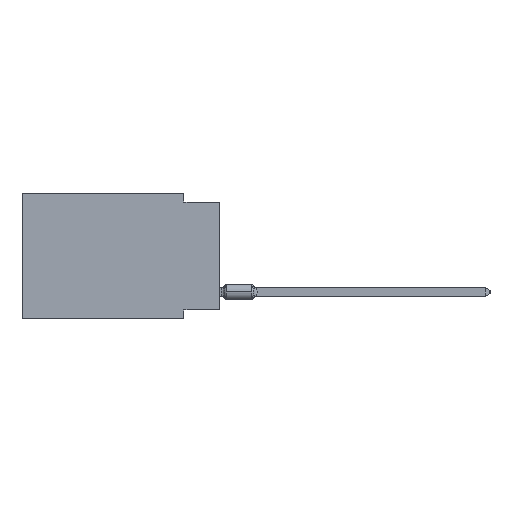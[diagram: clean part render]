
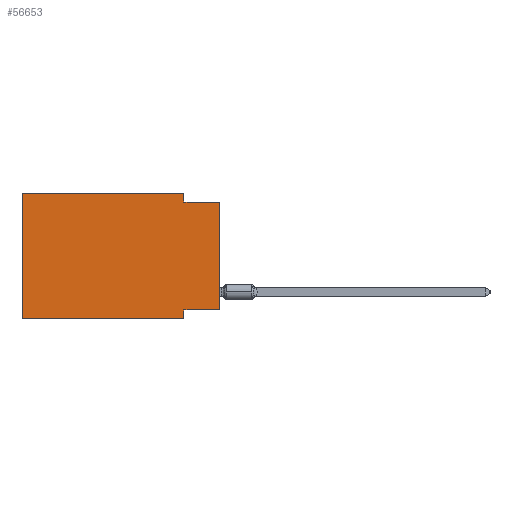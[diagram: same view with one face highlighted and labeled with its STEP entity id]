
A CAD part, left-side view. The second image highlights one B-rep face of the part: STEP entity #56653.
In plain terms, the highlighted planar face has unit normal (-1, 0, 0).
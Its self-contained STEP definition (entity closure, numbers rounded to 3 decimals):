
#1423 = ORIENTED_EDGE ( 'NONE', *, *, #35114, .F. ) ;
#5401 = CARTESIAN_POINT ( 'NONE',  ( 0., 13.97, 0. ) ) ;
#5918 = DIRECTION ( 'NONE',  ( 0., 0., 1. ) ) ;
#7233 = CARTESIAN_POINT ( 'NONE',  ( 0., 2.54, -8.255 ) ) ;
#7724 = LINE ( 'NONE', #23828, #65843 ) ;
#9683 = EDGE_CURVE ( 'NONE', #47627, #45161, #61070, .T. ) ;
#10409 = VERTEX_POINT ( 'NONE', #14607 ) ;
#11077 = ORIENTED_EDGE ( 'NONE', *, *, #18448, .F. ) ;
#14607 = CARTESIAN_POINT ( 'NONE',  ( 0., 0., -0.635 ) ) ;
#17439 = DIRECTION ( 'NONE',  ( 0., 0., 1. ) ) ;
#18448 = EDGE_CURVE ( 'NONE', #45444, #48281, #95899, .T. ) ;
#18705 = VECTOR ( 'NONE', #53018, 1000. ) ;
#22796 = CARTESIAN_POINT ( 'NONE',  ( 0., 2.54, -8.89 ) ) ;
#23828 = CARTESIAN_POINT ( 'NONE',  ( 0., 2.54, 0. ) ) ;
#24692 = VECTOR ( 'NONE', #36902, 1000. ) ;
#26858 = DIRECTION ( 'NONE',  ( 0., -1., 0. ) ) ;
#26885 = DIRECTION ( 'NONE',  ( 0., -1., 0. ) ) ;
#30345 = EDGE_CURVE ( 'NONE', #47627, #10409, #63252, .T. ) ;
#32315 = DIRECTION ( 'NONE',  ( 0., -1., 0. ) ) ;
#34377 = CARTESIAN_POINT ( 'NONE',  ( 0., 0., -0.635 ) ) ;
#35075 = VECTOR ( 'NONE', #26858, 1000. ) ;
#35114 = EDGE_CURVE ( 'NONE', #48281, #82652, #7724, .T. ) ;
#36902 = DIRECTION ( 'NONE',  ( 0., 1., 0. ) ) ;
#39866 = CARTESIAN_POINT ( 'NONE',  ( 0., 13.97, -8.89 ) ) ;
#41231 = ORIENTED_EDGE ( 'NONE', *, *, #56232, .T. ) ;
#42937 = VECTOR ( 'NONE', #17439, 1000. ) ;
#43924 = LINE ( 'NONE', #34377, #35075 ) ;
#45161 = VERTEX_POINT ( 'NONE', #7233 ) ;
#45444 = VERTEX_POINT ( 'NONE', #58999 ) ;
#47268 = ORIENTED_EDGE ( 'NONE', *, *, #9683, .F. ) ;
#47627 = VERTEX_POINT ( 'NONE', #49974 ) ;
#48281 = VERTEX_POINT ( 'NONE', #71784 ) ;
#49974 = CARTESIAN_POINT ( 'NONE',  ( 0., 0., -8.255 ) ) ;
#50646 = CARTESIAN_POINT ( 'NONE',  ( 0., 13.97, 0. ) ) ;
#53018 = DIRECTION ( 'NONE',  ( 0., 0., -1. ) ) ;
#53118 = CARTESIAN_POINT ( 'NONE',  ( 0., 13.97, -8.89 ) ) ;
#54215 = CARTESIAN_POINT ( 'NONE',  ( 0., 0., 0. ) ) ;
#56232 = EDGE_CURVE ( 'NONE', #90997, #75445, #63529, .T. ) ;
#56653 = ADVANCED_FACE ( 'NONE', ( #96994 ), #64756, .F. ) ;
#58999 = CARTESIAN_POINT ( 'NONE',  ( 0., 13.97, 0. ) ) ;
#59613 = ORIENTED_EDGE ( 'NONE', *, *, #30345, .T. ) ;
#60508 = ORIENTED_EDGE ( 'NONE', *, *, #86798, .F. ) ;
#61070 = LINE ( 'NONE', #89805, #24692 ) ;
#62747 = ORIENTED_EDGE ( 'NONE', *, *, #89873, .F. ) ;
#63252 = LINE ( 'NONE', #54215, #42937 ) ;
#63529 = LINE ( 'NONE', #39866, #83798 ) ;
#64756 = PLANE ( 'NONE',  #88687 ) ;
#65843 = VECTOR ( 'NONE', #91332, 1000. ) ;
#67819 = LINE ( 'NONE', #5401, #80966 ) ;
#70883 = CARTESIAN_POINT ( 'NONE',  ( 0., 2.54, -0.635 ) ) ;
#71784 = CARTESIAN_POINT ( 'NONE',  ( 0., 2.54, 0. ) ) ;
#72738 = ORIENTED_EDGE ( 'NONE', *, *, #81994, .F. ) ;
#75445 = VERTEX_POINT ( 'NONE', #79021 ) ;
#79021 = CARTESIAN_POINT ( 'NONE',  ( 0., 2.54, -8.89 ) ) ;
#79883 = DIRECTION ( 'NONE',  ( 0., 0., -1. ) ) ;
#80966 = VECTOR ( 'NONE', #5918, 1000. ) ;
#81994 = EDGE_CURVE ( 'NONE', #90997, #45444, #67819, .T. ) ;
#82652 = VERTEX_POINT ( 'NONE', #70883 ) ;
#83798 = VECTOR ( 'NONE', #32315, 1000. ) ;
#86798 = EDGE_CURVE ( 'NONE', #82652, #10409, #43924, .T. ) ;
#86959 = DIRECTION ( 'NONE',  ( 1., 0., 0. ) ) ;
#87332 = CARTESIAN_POINT ( 'NONE',  ( 0., 13.97, 0. ) ) ;
#88687 = AXIS2_PLACEMENT_3D ( 'NONE', #50646, #86959, #79883 ) ;
#89172 = EDGE_LOOP ( 'NONE', ( #59613, #60508, #1423, #11077, #72738, #41231, #62747, #47268 ) ) ;
#89805 = CARTESIAN_POINT ( 'NONE',  ( 0., 0., -8.255 ) ) ;
#89873 = EDGE_CURVE ( 'NONE', #45161, #75445, #91309, .T. ) ;
#90997 = VERTEX_POINT ( 'NONE', #53118 ) ;
#91309 = LINE ( 'NONE', #22796, #18705 ) ;
#91332 = DIRECTION ( 'NONE',  ( 0., 0., -1. ) ) ;
#95899 = LINE ( 'NONE', #87332, #97949 ) ;
#96994 = FACE_OUTER_BOUND ( 'NONE', #89172, .T. ) ;
#97949 = VECTOR ( 'NONE', #26885, 1000. ) ;
